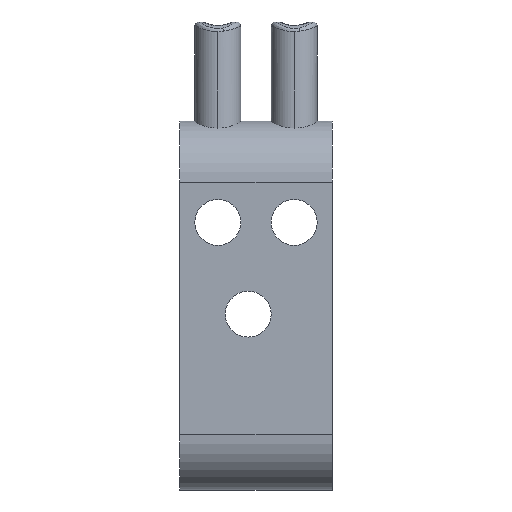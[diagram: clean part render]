
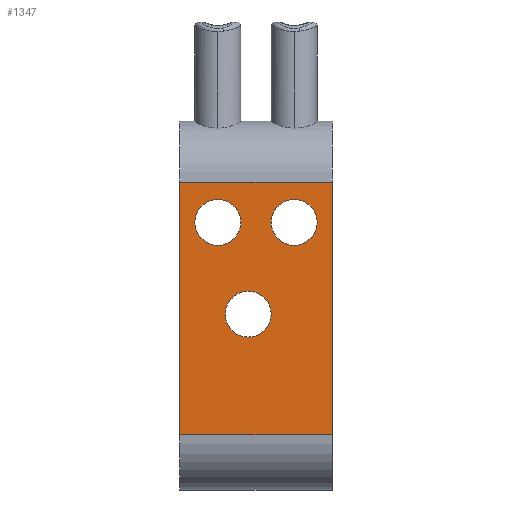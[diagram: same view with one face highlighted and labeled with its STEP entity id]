
A CAD part, left-side view. The second image highlights one B-rep face of the part: STEP entity #1347.
In plain terms, the highlighted planar face has unit normal (-1, 0, 0).
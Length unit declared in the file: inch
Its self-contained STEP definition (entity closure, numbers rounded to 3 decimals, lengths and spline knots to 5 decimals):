
#4 = LINE ( 'NONE', #146, #3953 ) ;
#5 = CARTESIAN_POINT ( 'NONE',  ( -0.28543, -0.19685, -1.32874 ) ) ;
#56 = DIRECTION ( 'NONE',  ( -1., 0., 0. ) ) ;
#103 = CARTESIAN_POINT ( 'NONE',  ( -0.28543, -0.19685, -1.32874 ) ) ;
#130 = ORIENTED_EDGE ( 'NONE', *, *, #2028, .F. ) ;
#143 = VECTOR ( 'NONE', #1434, 39.37008 ) ;
#146 = CARTESIAN_POINT ( 'NONE',  ( -0.28543, 0.59055, -0.62992 ) ) ;
#183 = CARTESIAN_POINT ( 'NONE',  ( -0.28543, 0.23708, -0.70866 ) ) ;
#237 = VERTEX_POINT ( 'NONE', #3380 ) ;
#273 = ORIENTED_EDGE ( 'NONE', *, *, #1602, .T. ) ;
#322 = VERTEX_POINT ( 'NONE', #1986 ) ;
#359 = CARTESIAN_POINT ( 'NONE',  ( -0.28543, 0.59055, -1.32874 ) ) ;
#381 = VERTEX_POINT ( 'NONE', #1418 ) ;
#456 = EDGE_CURVE ( 'NONE', #2228, #381, #4, .T. ) ;
#503 = DIRECTION ( 'NONE',  ( 0., 0., -1. ) ) ;
#504 = AXIS2_PLACEMENT_3D ( 'NONE', #183, #2404, #503 ) ;
#525 = EDGE_CURVE ( 'NONE', #237, #3027, #1887, .T. ) ;
#535 = ORIENTED_EDGE ( 'NONE', *, *, #2250, .F. ) ;
#539 = CIRCLE ( 'NONE', #504, 0.11811 ) ;
#551 = AXIS2_PLACEMENT_3D ( 'NONE', #2700, #813, #3012 ) ;
#554 = ORIENTED_EDGE ( 'NONE', *, *, #637, .F. ) ;
#606 = EDGE_CURVE ( 'NONE', #237, #381, #641, .T. ) ;
#628 = AXIS2_PLACEMENT_3D ( 'NONE', #1756, #3907, #2078 ) ;
#637 = EDGE_CURVE ( 'NONE', #1543, #1776, #1596, .T. ) ;
#641 = LINE ( 'NONE', #3894, #3863 ) ;
#657 = EDGE_CURVE ( 'NONE', #2424, #2064, #1498, .T. ) ;
#691 = VERTEX_POINT ( 'NONE', #1457 ) ;
#705 = EDGE_CURVE ( 'NONE', #691, #322, #539, .T. ) ;
#785 = DIRECTION ( 'NONE',  ( 0., 0., 1. ) ) ;
#813 = DIRECTION ( 'NONE',  ( -1., 0., 0. ) ) ;
#888 = ORIENTED_EDGE ( 'NONE', *, *, #525, .F. ) ;
#1036 = ORIENTED_EDGE ( 'NONE', *, *, #606, .T. ) ;
#1095 = DIRECTION ( 'NONE',  ( -1., 0., 0. ) ) ;
#1281 = CIRCLE ( 'NONE', #3013, 0.11811 ) ;
#1347 = ADVANCED_FACE ( 'NONE', ( #3138, #3848, #2316, #3044 ), #1739, .F. ) ;
#1395 = ORIENTED_EDGE ( 'NONE', *, *, #456, .F. ) ;
#1418 = CARTESIAN_POINT ( 'NONE',  ( -0.28543, 0.59055, -0.02953 ) ) ;
#1434 = DIRECTION ( 'NONE',  ( 0., -1., 0. ) ) ;
#1457 = CARTESIAN_POINT ( 'NONE',  ( -0.28543, 0.11897, -0.70866 ) ) ;
#1498 = CIRCLE ( 'NONE', #551, 0.11811 ) ;
#1539 = ORIENTED_EDGE ( 'NONE', *, *, #657, .F. ) ;
#1543 = VERTEX_POINT ( 'NONE', #2248 ) ;
#1596 = CIRCLE ( 'NONE', #628, 0.11811 ) ;
#1602 = EDGE_CURVE ( 'NONE', #2228, #3027, #1921, .T. ) ;
#1687 = EDGE_LOOP ( 'NONE', ( #3432, #3494 ) ) ;
#1739 = PLANE ( 'NONE',  #3156 ) ;
#1750 = DIRECTION ( 'NONE',  ( 1., 0., 0. ) ) ;
#1756 = CARTESIAN_POINT ( 'NONE',  ( -0.28543, 0., -0.23622 ) ) ;
#1757 = AXIS2_PLACEMENT_3D ( 'NONE', #1960, #56, #2273 ) ;
#1776 = VERTEX_POINT ( 'NONE', #3026 ) ;
#1833 = EDGE_CURVE ( 'NONE', #322, #691, #3222, .T. ) ;
#1869 = CARTESIAN_POINT ( 'NONE',  ( -0.28543, 0.23708, -0.70866 ) ) ;
#1887 = LINE ( 'NONE', #2674, #2335 ) ;
#1921 = LINE ( 'NONE', #103, #143 ) ;
#1960 = CARTESIAN_POINT ( 'NONE',  ( -0.28543, 0., -0.23622 ) ) ;
#1986 = CARTESIAN_POINT ( 'NONE',  ( -0.28543, 0.35519, -0.70866 ) ) ;
#2028 = EDGE_CURVE ( 'NONE', #2064, #2424, #1281, .T. ) ;
#2064 = VERTEX_POINT ( 'NONE', #2655 ) ;
#2078 = DIRECTION ( 'NONE',  ( 0., 0., 1. ) ) ;
#2180 = EDGE_LOOP ( 'NONE', ( #1539, #130 ) ) ;
#2194 = DIRECTION ( 'NONE',  ( 0., 0., -1. ) ) ;
#2228 = VERTEX_POINT ( 'NONE', #359 ) ;
#2248 = CARTESIAN_POINT ( 'NONE',  ( -0.28543, 0., -0.11811 ) ) ;
#2250 = EDGE_CURVE ( 'NONE', #1776, #1543, #2651, .T. ) ;
#2273 = DIRECTION ( 'NONE',  ( 0., 0., 1. ) ) ;
#2316 = FACE_BOUND ( 'NONE', #2180, .T. ) ;
#2335 = VECTOR ( 'NONE', #3603, 39.37008 ) ;
#2404 = DIRECTION ( 'NONE',  ( -1., 0., 0. ) ) ;
#2424 = VERTEX_POINT ( 'NONE', #4015 ) ;
#2651 = CIRCLE ( 'NONE', #1757, 0.11811 ) ;
#2655 = CARTESIAN_POINT ( 'NONE',  ( -0.28543, 0.3937, -0.35433 ) ) ;
#2674 = CARTESIAN_POINT ( 'NONE',  ( -0.28543, -0.19685, 0. ) ) ;
#2700 = CARTESIAN_POINT ( 'NONE',  ( -0.28543, 0.3937, -0.23622 ) ) ;
#2968 = CARTESIAN_POINT ( 'NONE',  ( -0.28543, 0.3937, -0.23622 ) ) ;
#2999 = DIRECTION ( 'NONE',  ( 0., 1., 0. ) ) ;
#3012 = DIRECTION ( 'NONE',  ( 0., 0., 1. ) ) ;
#3013 = AXIS2_PLACEMENT_3D ( 'NONE', #2968, #1095, #3274 ) ;
#3026 = CARTESIAN_POINT ( 'NONE',  ( -0.28543, 0., -0.35433 ) ) ;
#3027 = VERTEX_POINT ( 'NONE', #5 ) ;
#3044 = FACE_BOUND ( 'NONE', #1687, .T. ) ;
#3138 = FACE_OUTER_BOUND ( 'NONE', #3634, .T. ) ;
#3156 = AXIS2_PLACEMENT_3D ( 'NONE', #3611, #1750, #3902 ) ;
#3222 = CIRCLE ( 'NONE', #3576, 0.11811 ) ;
#3274 = DIRECTION ( 'NONE',  ( 0., 0., 1. ) ) ;
#3380 = CARTESIAN_POINT ( 'NONE',  ( -0.28543, -0.19685, -0.02953 ) ) ;
#3432 = ORIENTED_EDGE ( 'NONE', *, *, #705, .F. ) ;
#3494 = ORIENTED_EDGE ( 'NONE', *, *, #1833, .F. ) ;
#3576 = AXIS2_PLACEMENT_3D ( 'NONE', #1869, #4023, #2194 ) ;
#3603 = DIRECTION ( 'NONE',  ( 0., 0., -1. ) ) ;
#3611 = CARTESIAN_POINT ( 'NONE',  ( -0.28543, -0.11811, -0.98425 ) ) ;
#3634 = EDGE_LOOP ( 'NONE', ( #1395, #273, #888, #1036 ) ) ;
#3718 = EDGE_LOOP ( 'NONE', ( #554, #535 ) ) ;
#3848 = FACE_BOUND ( 'NONE', #3718, .T. ) ;
#3863 = VECTOR ( 'NONE', #2999, 39.37008 ) ;
#3894 = CARTESIAN_POINT ( 'NONE',  ( -0.28543, 0.59055, -0.02953 ) ) ;
#3902 = DIRECTION ( 'NONE',  ( 0., 0., -1. ) ) ;
#3907 = DIRECTION ( 'NONE',  ( -1., 0., 0. ) ) ;
#3953 = VECTOR ( 'NONE', #785, 39.37008 ) ;
#4015 = CARTESIAN_POINT ( 'NONE',  ( -0.28543, 0.3937, -0.11811 ) ) ;
#4023 = DIRECTION ( 'NONE',  ( -1., 0., 0. ) ) ;
